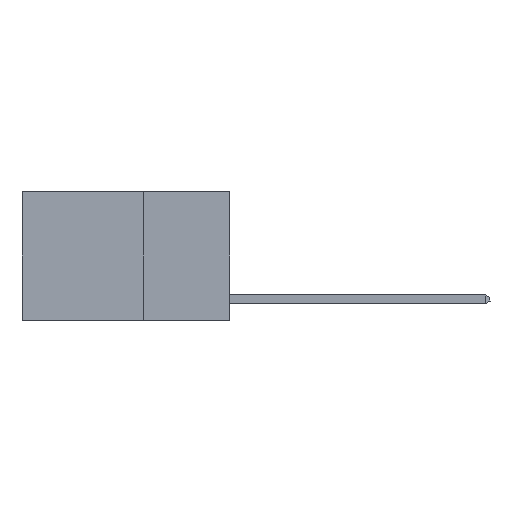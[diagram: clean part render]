
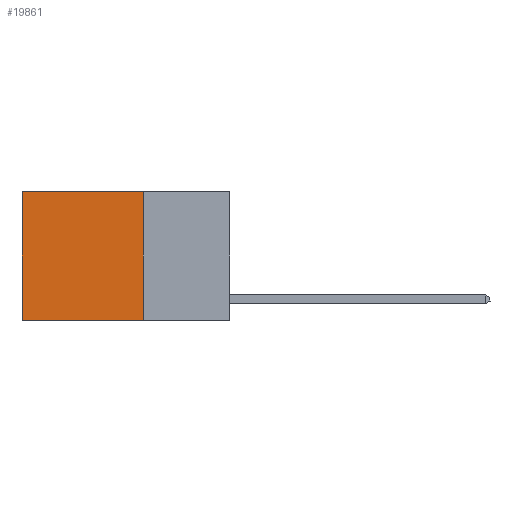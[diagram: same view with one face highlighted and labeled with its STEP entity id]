
A CAD part, left-side view. The second image highlights one B-rep face of the part: STEP entity #19861.
In plain terms, the highlighted planar face has unit normal (-1, 0, 0).
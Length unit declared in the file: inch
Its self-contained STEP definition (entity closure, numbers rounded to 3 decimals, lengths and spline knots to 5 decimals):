
#234 = ORIENTED_EDGE ( 'NONE', *, *, #9912, .T. ) ;
#309 = FACE_OUTER_BOUND ( 'NONE', #5966, .T. ) ;
#320 = CARTESIAN_POINT ( 'NONE',  ( 0.2625, 0.6, -0.37 ) ) ;
#961 = CARTESIAN_POINT ( 'NONE',  ( 0.2625, 0.6, 0. ) ) ;
#1945 = EDGE_CURVE ( 'NONE', #9663, #9564, #16181, .T. ) ;
#2012 = DIRECTION ( 'NONE',  ( 1., 0., 0. ) ) ;
#2528 = VERTEX_POINT ( 'NONE', #320 ) ;
#3262 = CARTESIAN_POINT ( 'NONE',  ( 0.2625, 0.6, 0. ) ) ;
#4121 = ORIENTED_EDGE ( 'NONE', *, *, #18185, .T. ) ;
#4794 = CARTESIAN_POINT ( 'NONE',  ( 0.2625, 0.25, 0. ) ) ;
#5959 = ORIENTED_EDGE ( 'NONE', *, *, #1945, .F. ) ;
#5966 = EDGE_LOOP ( 'NONE', ( #234, #13386, #5959, #4121 ) ) ;
#6320 = DIRECTION ( 'NONE',  ( 0., 0., -1. ) ) ;
#6508 = DIRECTION ( 'NONE',  ( 0., 1., 0. ) ) ;
#7529 = CARTESIAN_POINT ( 'NONE',  ( 0.2625, 0.25, -0.37 ) ) ;
#7653 = VECTOR ( 'NONE', #20005, 39.37008 ) ;
#7923 = EDGE_CURVE ( 'NONE', #9564, #2528, #13434, .T. ) ;
#9449 = CARTESIAN_POINT ( 'NONE',  ( 0.2625, 0.25, 0. ) ) ;
#9564 = VERTEX_POINT ( 'NONE', #7529 ) ;
#9663 = VERTEX_POINT ( 'NONE', #15993 ) ;
#9789 = DIRECTION ( 'NONE',  ( 0., 0., -1. ) ) ;
#9912 = EDGE_CURVE ( 'NONE', #18498, #2528, #19536, .T. ) ;
#11313 = DIRECTION ( 'NONE',  ( 0., 0., -1. ) ) ;
#12948 = CARTESIAN_POINT ( 'NONE',  ( 0.2625, 0.25, 0. ) ) ;
#13386 = ORIENTED_EDGE ( 'NONE', *, *, #7923, .F. ) ;
#13434 = LINE ( 'NONE', #16786, #7653 ) ;
#14741 = VECTOR ( 'NONE', #6320, 39.37008 ) ;
#14847 = PLANE ( 'NONE',  #15960 ) ;
#15960 = AXIS2_PLACEMENT_3D ( 'NONE', #4794, #2012, #11313 ) ;
#15993 = CARTESIAN_POINT ( 'NONE',  ( 0.2625, 0.25, 0. ) ) ;
#16181 = LINE ( 'NONE', #9449, #14741 ) ;
#16786 = CARTESIAN_POINT ( 'NONE',  ( 0.2625, 0.25, -0.37 ) ) ;
#18185 = EDGE_CURVE ( 'NONE', #9663, #18498, #18206, .T. ) ;
#18206 = LINE ( 'NONE', #12948, #18657 ) ;
#18498 = VERTEX_POINT ( 'NONE', #961 ) ;
#18657 = VECTOR ( 'NONE', #6508, 39.37008 ) ;
#19229 = VECTOR ( 'NONE', #9789, 39.37008 ) ;
#19536 = LINE ( 'NONE', #3262, #19229 ) ;
#19861 = ADVANCED_FACE ( 'NONE', ( #309 ), #14847, .F. ) ;
#20005 = DIRECTION ( 'NONE',  ( 0., 1., 0. ) ) ;
